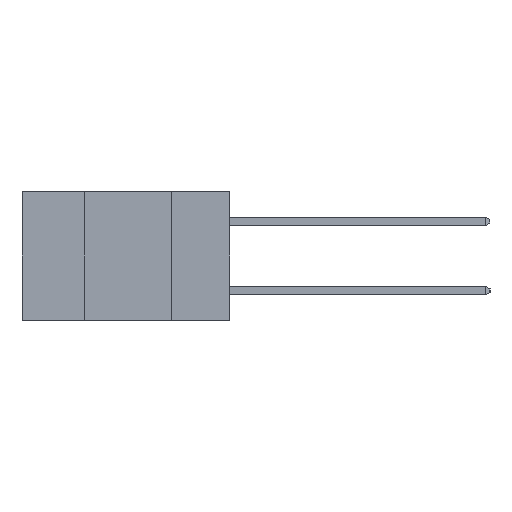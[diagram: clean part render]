
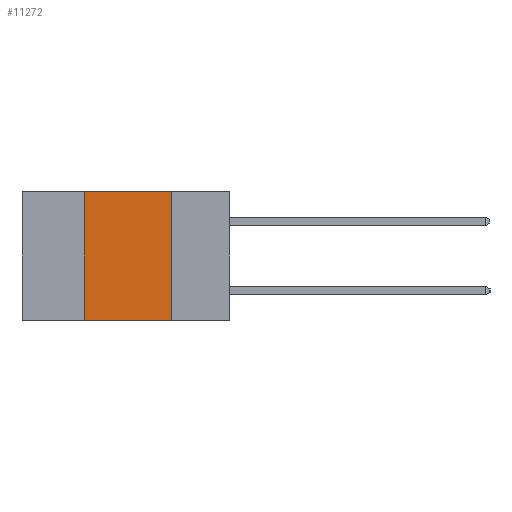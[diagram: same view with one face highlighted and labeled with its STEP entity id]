
A CAD part, left-side view. The second image highlights one B-rep face of the part: STEP entity #11272.
In plain terms, the highlighted planar face has unit normal (-1, 0, 0).
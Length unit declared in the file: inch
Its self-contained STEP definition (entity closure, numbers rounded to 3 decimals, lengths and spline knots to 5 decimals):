
#1808 = CARTESIAN_POINT ( 'NONE',  ( 0., 0.17, -0.37 ) ) ;
#2395 = CARTESIAN_POINT ( 'NONE',  ( 0., 0.42, 0. ) ) ;
#3143 = VECTOR ( 'NONE', #5541, 39.37008 ) ;
#3410 = CARTESIAN_POINT ( 'NONE',  ( 0., 0.6, 0. ) ) ;
#3839 = VERTEX_POINT ( 'NONE', #16318 ) ;
#3983 = EDGE_LOOP ( 'NONE', ( #19172, #14109, #17522, #8851 ) ) ;
#5541 = DIRECTION ( 'NONE',  ( 0., -1., 0. ) ) ;
#6256 = CARTESIAN_POINT ( 'NONE',  ( 0., 0.6, -0.37 ) ) ;
#7186 = AXIS2_PLACEMENT_3D ( 'NONE', #3410, #20954, #10477 ) ;
#7235 = CARTESIAN_POINT ( 'NONE',  ( 0., 0.6, 0. ) ) ;
#8851 = ORIENTED_EDGE ( 'NONE', *, *, #9084, .T. ) ;
#9084 = EDGE_CURVE ( 'NONE', #3839, #19891, #20235, .T. ) ;
#9518 = DIRECTION ( 'NONE',  ( 0., 0., 1. ) ) ;
#9786 = DIRECTION ( 'NONE',  ( 0., -1., 0. ) ) ;
#10270 = EDGE_CURVE ( 'NONE', #3839, #21497, #16357, .T. ) ;
#10477 = DIRECTION ( 'NONE',  ( 0., 0., -1. ) ) ;
#11100 = FACE_OUTER_BOUND ( 'NONE', #3983, .T. ) ;
#11259 = CARTESIAN_POINT ( 'NONE',  ( 0., 0.17, -0.37 ) ) ;
#11272 = ADVANCED_FACE ( 'NONE', ( #11100 ), #13928, .F. ) ;
#11436 = EDGE_CURVE ( 'NONE', #21497, #18951, #13035, .T. ) ;
#13035 = LINE ( 'NONE', #7235, #3143 ) ;
#13113 = DIRECTION ( 'NONE',  ( 0., 0., -1. ) ) ;
#13797 = EDGE_CURVE ( 'NONE', #18951, #19891, #20887, .T. ) ;
#13928 = PLANE ( 'NONE',  #7186 ) ;
#14109 = ORIENTED_EDGE ( 'NONE', *, *, #11436, .F. ) ;
#14701 = VECTOR ( 'NONE', #9518, 39.37008 ) ;
#16236 = VECTOR ( 'NONE', #13113, 39.37008 ) ;
#16318 = CARTESIAN_POINT ( 'NONE',  ( 0., 0.42, -0.37 ) ) ;
#16357 = LINE ( 'NONE', #21733, #14701 ) ;
#17522 = ORIENTED_EDGE ( 'NONE', *, *, #10270, .F. ) ;
#18301 = CARTESIAN_POINT ( 'NONE',  ( 0., 0.17, 0. ) ) ;
#18951 = VERTEX_POINT ( 'NONE', #18301 ) ;
#19172 = ORIENTED_EDGE ( 'NONE', *, *, #13797, .F. ) ;
#19680 = VECTOR ( 'NONE', #9786, 39.37008 ) ;
#19891 = VERTEX_POINT ( 'NONE', #1808 ) ;
#20235 = LINE ( 'NONE', #6256, #19680 ) ;
#20887 = LINE ( 'NONE', #11259, #16236 ) ;
#20954 = DIRECTION ( 'NONE',  ( 1., 0., 0. ) ) ;
#21497 = VERTEX_POINT ( 'NONE', #2395 ) ;
#21733 = CARTESIAN_POINT ( 'NONE',  ( 0., 0.42, -0.37 ) ) ;
